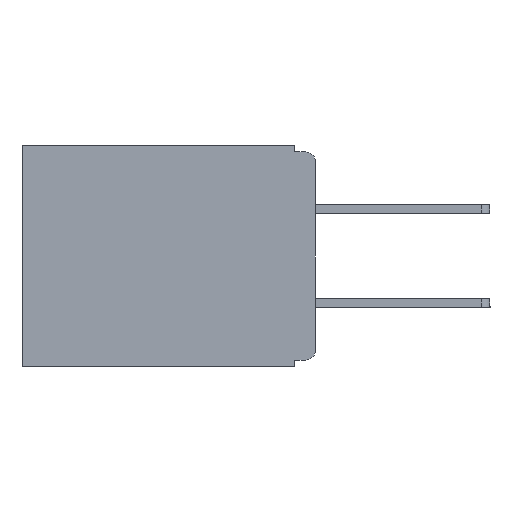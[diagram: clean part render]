
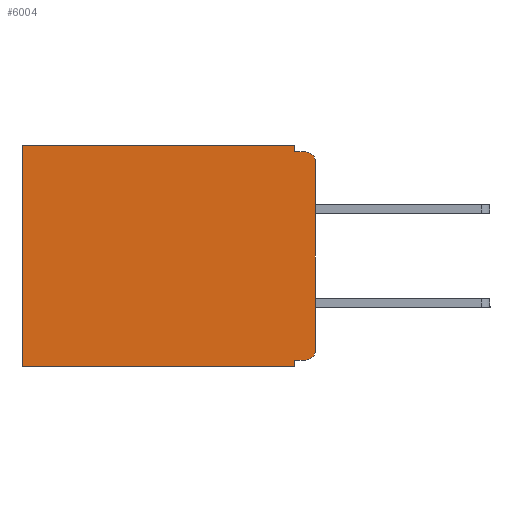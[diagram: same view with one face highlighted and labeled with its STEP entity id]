
A CAD part, left-side view. The second image highlights one B-rep face of the part: STEP entity #6004.
In plain terms, the highlighted planar face has unit normal (-1, 0, 0).
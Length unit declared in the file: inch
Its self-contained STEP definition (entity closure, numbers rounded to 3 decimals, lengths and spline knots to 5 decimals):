
#208 = VECTOR ( 'NONE', #9866, 39.37008 ) ;
#577 = ORIENTED_EDGE ( 'NONE', *, *, #11478, .T. ) ;
#1031 = DIRECTION ( 'NONE',  ( 0., 0., -1. ) ) ;
#1248 = AXIS2_PLACEMENT_3D ( 'NONE', #2258, #12216, #3718 ) ;
#1278 = VERTEX_POINT ( 'NONE', #16521 ) ;
#1333 = VERTEX_POINT ( 'NONE', #14418 ) ;
#1369 = LINE ( 'NONE', #14601, #5235 ) ;
#1482 = ORIENTED_EDGE ( 'NONE', *, *, #11589, .F. ) ;
#1733 = ORIENTED_EDGE ( 'NONE', *, *, #2588, .F. ) ;
#1850 = VERTEX_POINT ( 'NONE', #10591 ) ;
#1876 = VERTEX_POINT ( 'NONE', #8714 ) ;
#1907 = EDGE_LOOP ( 'NONE', ( #1733, #577, #3766, #1482, #12813, #2412, #5884, #8868, #6279, #14558 ) ) ;
#2258 = CARTESIAN_POINT ( 'NONE',  ( 0.3, 0.015, -0.025 ) ) ;
#2412 = ORIENTED_EDGE ( 'NONE', *, *, #11452, .T. ) ;
#2583 = VERTEX_POINT ( 'NONE', #17125 ) ;
#2588 = EDGE_CURVE ( 'NONE', #1278, #1850, #11108, .T. ) ;
#2615 = CARTESIAN_POINT ( 'NONE',  ( 0.3, 0., -0.33 ) ) ;
#2729 = CIRCLE ( 'NONE', #1248, 0.015 ) ;
#3332 = DIRECTION ( 'NONE',  ( 0., -1., 0. ) ) ;
#3718 = DIRECTION ( 'NONE',  ( 0., 0., -1. ) ) ;
#3729 = CARTESIAN_POINT ( 'NONE',  ( 0.3, 0.031, -0.33 ) ) ;
#3766 = ORIENTED_EDGE ( 'NONE', *, *, #10166, .F. ) ;
#4081 = LINE ( 'NONE', #2615, #11158 ) ;
#4351 = EDGE_CURVE ( 'NONE', #2583, #5982, #1369, .T. ) ;
#5041 = CARTESIAN_POINT ( 'NONE',  ( 0.3, 0.437, -0.33 ) ) ;
#5075 = EDGE_CURVE ( 'NONE', #1333, #2583, #11173, .T. ) ;
#5106 = DIRECTION ( 'NONE',  ( 1., 0., 0. ) ) ;
#5235 = VECTOR ( 'NONE', #14181, 39.37008 ) ;
#5253 = VECTOR ( 'NONE', #3332, 39.37008 ) ;
#5495 = CARTESIAN_POINT ( 'NONE',  ( 0.3, 0.015, -0.01 ) ) ;
#5884 = ORIENTED_EDGE ( 'NONE', *, *, #12506, .F. ) ;
#5982 = VERTEX_POINT ( 'NONE', #3729 ) ;
#6004 = ADVANCED_FACE ( 'NONE', ( #18040 ), #15138, .F. ) ;
#6150 = CARTESIAN_POINT ( 'NONE',  ( 0.3, 0., -0.33 ) ) ;
#6202 = DIRECTION ( 'NONE',  ( -1., 0., 0. ) ) ;
#6279 = ORIENTED_EDGE ( 'NONE', *, *, #5075, .F. ) ;
#6758 = CIRCLE ( 'NONE', #9424, 0.015 ) ;
#6998 = VECTOR ( 'NONE', #9228, 39.37008 ) ;
#7044 = EDGE_CURVE ( 'NONE', #1876, #8321, #9319, .T. ) ;
#7908 = VECTOR ( 'NONE', #1031, 39.37008 ) ;
#8169 = CARTESIAN_POINT ( 'NONE',  ( 0.3, 0.437, -0.33 ) ) ;
#8321 = VERTEX_POINT ( 'NONE', #11297 ) ;
#8609 = VERTEX_POINT ( 'NONE', #8169 ) ;
#8714 = CARTESIAN_POINT ( 'NONE',  ( 0.3, 0.031, 0. ) ) ;
#8868 = ORIENTED_EDGE ( 'NONE', *, *, #4351, .F. ) ;
#8967 = CARTESIAN_POINT ( 'NONE',  ( 0.3, 0., -0.33 ) ) ;
#8987 = LINE ( 'NONE', #17307, #5253 ) ;
#9228 = DIRECTION ( 'NONE',  ( 0., 0., -1. ) ) ;
#9319 = LINE ( 'NONE', #14654, #12215 ) ;
#9424 = AXIS2_PLACEMENT_3D ( 'NONE', #14674, #6202, #16036 ) ;
#9788 = CARTESIAN_POINT ( 'NONE',  ( 0.3, 0., -0.32 ) ) ;
#9866 = DIRECTION ( 'NONE',  ( 0., 1., 0. ) ) ;
#10166 = EDGE_CURVE ( 'NONE', #11398, #15017, #8987, .T. ) ;
#10263 = LINE ( 'NONE', #5041, #6998 ) ;
#10591 = CARTESIAN_POINT ( 'NONE',  ( 0.3, 0., -0.305 ) ) ;
#10990 = AXIS2_PLACEMENT_3D ( 'NONE', #6150, #5106, #12193 ) ;
#11108 = LINE ( 'NONE', #8967, #15320 ) ;
#11136 = DIRECTION ( 'NONE',  ( 0., 1., 0. ) ) ;
#11158 = VECTOR ( 'NONE', #11136, 39.37008 ) ;
#11173 = LINE ( 'NONE', #9788, #208 ) ;
#11297 = CARTESIAN_POINT ( 'NONE',  ( 0.3, 0.437, 0. ) ) ;
#11398 = VERTEX_POINT ( 'NONE', #14833 ) ;
#11452 = EDGE_CURVE ( 'NONE', #8321, #8609, #10263, .T. ) ;
#11478 = EDGE_CURVE ( 'NONE', #1278, #15017, #2729, .T. ) ;
#11589 = EDGE_CURVE ( 'NONE', #1876, #11398, #11639, .T. ) ;
#11639 = LINE ( 'NONE', #15239, #7908 ) ;
#12193 = DIRECTION ( 'NONE',  ( 0., 0., -1. ) ) ;
#12215 = VECTOR ( 'NONE', #14211, 39.37008 ) ;
#12216 = DIRECTION ( 'NONE',  ( -1., 0., 0. ) ) ;
#12506 = EDGE_CURVE ( 'NONE', #5982, #8609, #4081, .T. ) ;
#12812 = EDGE_CURVE ( 'NONE', #1333, #1850, #6758, .T. ) ;
#12813 = ORIENTED_EDGE ( 'NONE', *, *, #7044, .T. ) ;
#14181 = DIRECTION ( 'NONE',  ( 0., 0., -1. ) ) ;
#14211 = DIRECTION ( 'NONE',  ( 0., 1., 0. ) ) ;
#14418 = CARTESIAN_POINT ( 'NONE',  ( 0.3, 0.015, -0.32 ) ) ;
#14558 = ORIENTED_EDGE ( 'NONE', *, *, #12812, .T. ) ;
#14601 = CARTESIAN_POINT ( 'NONE',  ( 0.3, 0.031, -0.33 ) ) ;
#14654 = CARTESIAN_POINT ( 'NONE',  ( 0.3, 0., 0. ) ) ;
#14674 = CARTESIAN_POINT ( 'NONE',  ( 0.3, 0.015, -0.305 ) ) ;
#14833 = CARTESIAN_POINT ( 'NONE',  ( 0.3, 0.031, -0.01 ) ) ;
#15017 = VERTEX_POINT ( 'NONE', #5495 ) ;
#15138 = PLANE ( 'NONE',  #10990 ) ;
#15239 = CARTESIAN_POINT ( 'NONE',  ( 0.3, 0.031, 0. ) ) ;
#15320 = VECTOR ( 'NONE', #16838, 39.37008 ) ;
#16036 = DIRECTION ( 'NONE',  ( 0., 0., -1. ) ) ;
#16521 = CARTESIAN_POINT ( 'NONE',  ( 0.3, 0., -0.025 ) ) ;
#16838 = DIRECTION ( 'NONE',  ( 0., 0., -1. ) ) ;
#17125 = CARTESIAN_POINT ( 'NONE',  ( 0.3, 0.031, -0.32 ) ) ;
#17307 = CARTESIAN_POINT ( 'NONE',  ( 0.3, 0., -0.01 ) ) ;
#18040 = FACE_OUTER_BOUND ( 'NONE', #1907, .T. ) ;
